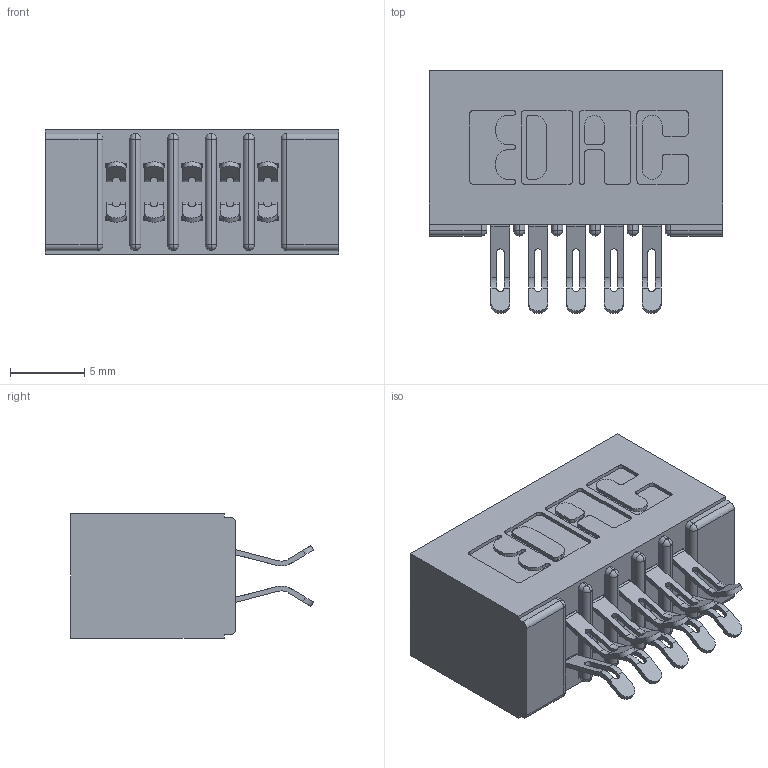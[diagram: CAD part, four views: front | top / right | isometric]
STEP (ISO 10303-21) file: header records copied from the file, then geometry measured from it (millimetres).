
FILE_DESCRIPTION (( 'STEP AP203' ), '1' );
FILE_NAME ('341-010-555-201.STEP', '2019-08-09T16:33:24', ( '' ), ( '' ), 'SwSTEP 2.0', 'SolidWorks 2016', '' );
FILE_SCHEMA (( 'CONFIG_CONTROL_DESIGN' ));
Length unit declared in the file: inch
Products named in the file (3): 341-010-555-201; 341-292-001_341-292-155; 341 Part_No Mounting Lugs
Assembly tree (11 placements, depth 2):
  341-010-555-201
    341 Part_No Mounting Lugs
    341-292-001_341-292-155  x10
Bounding box: 19.68 x 16.31 x 8.38 mm (x, y, z)
Volume: 1308.6 mm3; surface area: 2432.8 mm2
Topology: 11 solids, 11 shells, 888 faces, 2627 edges, 1710 vertices
Faces by surface type: plane 484, cylinder 384, sphere 12, torus 8
Entity records: 11172 total; most frequent: CARTESIAN_POINT 1873, ORIENTED_EDGE 1846, DIRECTION 1833, EDGE_CURVE 923, VECTOR 693, LINE 693, VERTEX_POINT 594, AXIS2_PLACEMENT_3D 570
